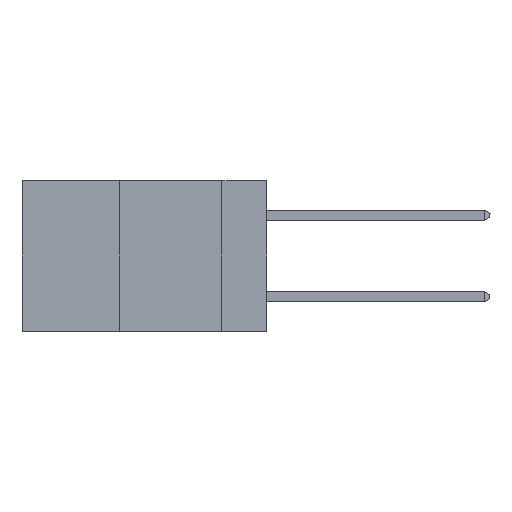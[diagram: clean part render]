
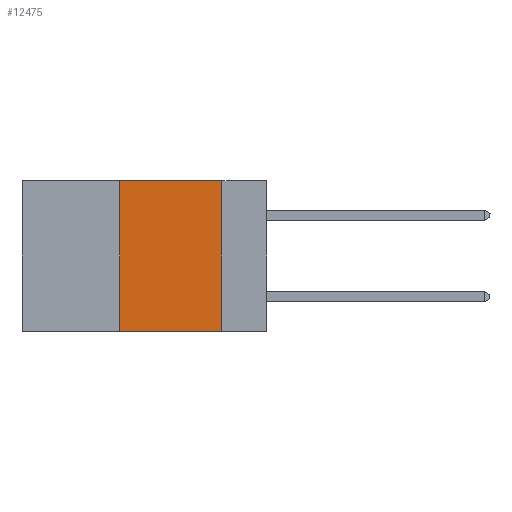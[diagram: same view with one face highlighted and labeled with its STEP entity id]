
A CAD part, left-side view. The second image highlights one B-rep face of the part: STEP entity #12475.
In plain terms, the highlighted planar face has unit normal (-1, 0, 0).
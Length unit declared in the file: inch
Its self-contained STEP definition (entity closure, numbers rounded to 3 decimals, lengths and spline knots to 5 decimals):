
#936 = EDGE_CURVE ( 'NONE', #13741, #7504, #13194, .T. ) ;
#2354 = EDGE_LOOP ( 'NONE', ( #10385, #10562, #14130, #10101 ) ) ;
#2920 = CARTESIAN_POINT ( 'NONE',  ( 0., 0.11, 0. ) ) ;
#2946 = AXIS2_PLACEMENT_3D ( 'NONE', #5272, #13571, #7400 ) ;
#2957 = LINE ( 'NONE', #7874, #11046 ) ;
#3534 = FACE_OUTER_BOUND ( 'NONE', #2354, .T. ) ;
#4050 = VERTEX_POINT ( 'NONE', #2920 ) ;
#4891 = VECTOR ( 'NONE', #13211, 39.37008 ) ;
#4920 = CARTESIAN_POINT ( 'NONE',  ( 0., 0.6, 0. ) ) ;
#5272 = CARTESIAN_POINT ( 'NONE',  ( 0., 0.6, 0. ) ) ;
#6567 = VECTOR ( 'NONE', #11298, 39.37008 ) ;
#7400 = DIRECTION ( 'NONE',  ( 0., 0., -1. ) ) ;
#7504 = VERTEX_POINT ( 'NONE', #11062 ) ;
#7874 = CARTESIAN_POINT ( 'NONE',  ( 0., 0.6, -0.37 ) ) ;
#9326 = VERTEX_POINT ( 'NONE', #12093 ) ;
#9795 = LINE ( 'NONE', #4920, #6567 ) ;
#10101 = ORIENTED_EDGE ( 'NONE', *, *, #12837, .T. ) ;
#10385 = ORIENTED_EDGE ( 'NONE', *, *, #11890, .F. ) ;
#10392 = VECTOR ( 'NONE', #12684, 39.37008 ) ;
#10562 = ORIENTED_EDGE ( 'NONE', *, *, #10946, .F. ) ;
#10653 = CARTESIAN_POINT ( 'NONE',  ( 0., 0.36, 0. ) ) ;
#10946 = EDGE_CURVE ( 'NONE', #7504, #4050, #9795, .T. ) ;
#11046 = VECTOR ( 'NONE', #14057, 39.37008 ) ;
#11062 = CARTESIAN_POINT ( 'NONE',  ( 0., 0.36, 0. ) ) ;
#11298 = DIRECTION ( 'NONE',  ( 0., -1., 0. ) ) ;
#11707 = CARTESIAN_POINT ( 'NONE',  ( 0., 0.11, 0. ) ) ;
#11890 = EDGE_CURVE ( 'NONE', #4050, #9326, #13027, .T. ) ;
#12093 = CARTESIAN_POINT ( 'NONE',  ( 0., 0.11, -0.37 ) ) ;
#12475 = ADVANCED_FACE ( 'NONE', ( #3534 ), #12571, .F. ) ;
#12571 = PLANE ( 'NONE',  #2946 ) ;
#12684 = DIRECTION ( 'NONE',  ( 0., 0., -1. ) ) ;
#12837 = EDGE_CURVE ( 'NONE', #13741, #9326, #2957, .T. ) ;
#13027 = LINE ( 'NONE', #11707, #10392 ) ;
#13194 = LINE ( 'NONE', #10653, #4891 ) ;
#13211 = DIRECTION ( 'NONE',  ( 0., 0., 1. ) ) ;
#13571 = DIRECTION ( 'NONE',  ( 1., 0., 0. ) ) ;
#13741 = VERTEX_POINT ( 'NONE', #14121 ) ;
#14057 = DIRECTION ( 'NONE',  ( 0., -1., 0. ) ) ;
#14121 = CARTESIAN_POINT ( 'NONE',  ( 0., 0.36, -0.37 ) ) ;
#14130 = ORIENTED_EDGE ( 'NONE', *, *, #936, .F. ) ;
